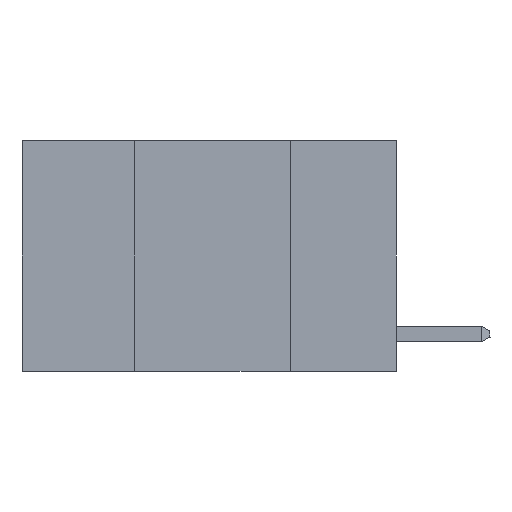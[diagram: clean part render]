
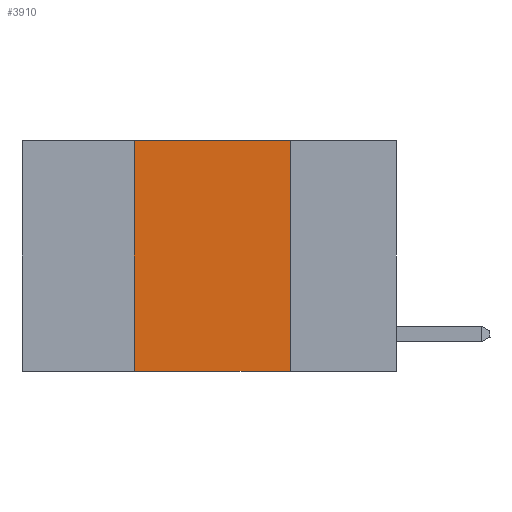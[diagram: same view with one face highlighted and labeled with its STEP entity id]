
A CAD part, left-side view. The second image highlights one B-rep face of the part: STEP entity #3910.
In plain terms, the highlighted planar face has unit normal (-1, 0, 0).
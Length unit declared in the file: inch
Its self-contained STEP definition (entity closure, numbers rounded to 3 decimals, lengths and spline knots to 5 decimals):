
#8 = FACE_OUTER_BOUND ( 'NONE', #15420, .T. ) ;
#362 = CARTESIAN_POINT ( 'NONE',  ( 0., 0.6, -0.37 ) ) ;
#496 = ORIENTED_EDGE ( 'NONE', *, *, #10452, .F. ) ;
#540 = VECTOR ( 'NONE', #13976, 39.37008 ) ;
#961 = AXIS2_PLACEMENT_3D ( 'NONE', #6148, #8691, #3763 ) ;
#1066 = VERTEX_POINT ( 'NONE', #11396 ) ;
#1583 = ORIENTED_EDGE ( 'NONE', *, *, #3460, .F. ) ;
#1591 = EDGE_CURVE ( 'NONE', #11087, #1066, #11461, .T. ) ;
#1797 = ORIENTED_EDGE ( 'NONE', *, *, #1591, .T. ) ;
#1993 = ORIENTED_EDGE ( 'NONE', *, *, #16020, .F. ) ;
#2337 = LINE ( 'NONE', #7363, #7584 ) ;
#3145 = VECTOR ( 'NONE', #6319, 39.37008 ) ;
#3460 = EDGE_CURVE ( 'NONE', #9704, #1066, #5858, .T. ) ;
#3763 = DIRECTION ( 'NONE',  ( 0., 0., -1. ) ) ;
#3910 = ADVANCED_FACE ( 'NONE', ( #8 ), #14849, .F. ) ;
#4251 = CARTESIAN_POINT ( 'NONE',  ( 0., 0.17, 0. ) ) ;
#5702 = CARTESIAN_POINT ( 'NONE',  ( 0., 0.17, 0. ) ) ;
#5858 = LINE ( 'NONE', #5702, #14318 ) ;
#6148 = CARTESIAN_POINT ( 'NONE',  ( 0., 0.6, 0. ) ) ;
#6319 = DIRECTION ( 'NONE',  ( 0., 0., 1. ) ) ;
#7363 = CARTESIAN_POINT ( 'NONE',  ( 0., 0.6, 0. ) ) ;
#7584 = VECTOR ( 'NONE', #8732, 39.37008 ) ;
#7941 = CARTESIAN_POINT ( 'NONE',  ( 0., 0.42, -0.37 ) ) ;
#8691 = DIRECTION ( 'NONE',  ( 1., 0., 0. ) ) ;
#8732 = DIRECTION ( 'NONE',  ( 0., -1., 0. ) ) ;
#9704 = VERTEX_POINT ( 'NONE', #4251 ) ;
#10091 = VERTEX_POINT ( 'NONE', #11354 ) ;
#10265 = CARTESIAN_POINT ( 'NONE',  ( 0., 0.42, 0. ) ) ;
#10452 = EDGE_CURVE ( 'NONE', #11087, #10091, #11498, .T. ) ;
#10868 = DIRECTION ( 'NONE',  ( 0., 0., -1. ) ) ;
#11087 = VERTEX_POINT ( 'NONE', #7941 ) ;
#11354 = CARTESIAN_POINT ( 'NONE',  ( 0., 0.42, 0. ) ) ;
#11396 = CARTESIAN_POINT ( 'NONE',  ( 0., 0.17, -0.37 ) ) ;
#11461 = LINE ( 'NONE', #362, #540 ) ;
#11498 = LINE ( 'NONE', #10265, #3145 ) ;
#13976 = DIRECTION ( 'NONE',  ( 0., -1., 0. ) ) ;
#14318 = VECTOR ( 'NONE', #10868, 39.37008 ) ;
#14849 = PLANE ( 'NONE',  #961 ) ;
#15420 = EDGE_LOOP ( 'NONE', ( #1583, #1993, #496, #1797 ) ) ;
#16020 = EDGE_CURVE ( 'NONE', #10091, #9704, #2337, .T. ) ;
